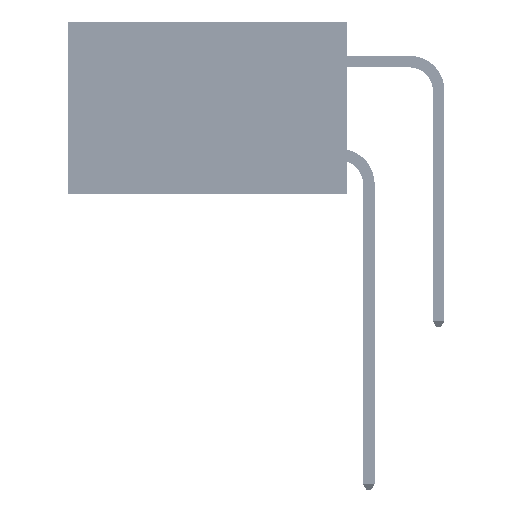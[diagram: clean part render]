
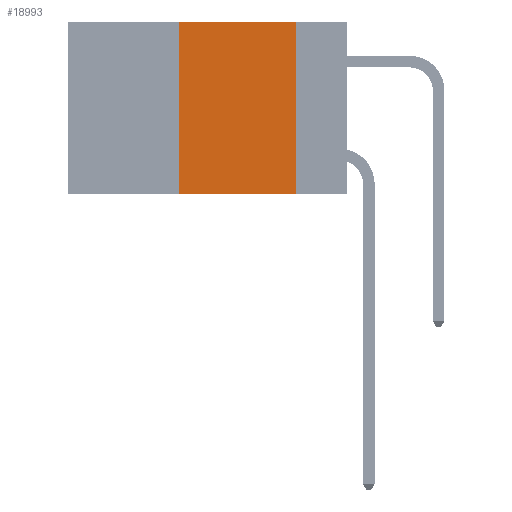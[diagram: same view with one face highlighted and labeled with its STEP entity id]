
A CAD part, left-side view. The second image highlights one B-rep face of the part: STEP entity #18993.
In plain terms, the highlighted planar face has unit normal (-1, 0, 0).
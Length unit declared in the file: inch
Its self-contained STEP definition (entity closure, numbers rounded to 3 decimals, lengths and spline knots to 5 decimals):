
#2547 = LINE ( 'NONE', #6751, #9694 ) ;
#3006 = LINE ( 'NONE', #51814, #30698 ) ;
#5474 = DIRECTION ( 'NONE',  ( 0., 0., -1. ) ) ;
#6481 = LINE ( 'NONE', #18073, #32411 ) ;
#6751 = CARTESIAN_POINT ( 'NONE',  ( 0., 0.36, 0. ) ) ;
#9428 = FACE_OUTER_BOUND ( 'NONE', #39500, .T. ) ;
#9694 = VECTOR ( 'NONE', #34959, 39.37008 ) ;
#10251 = ORIENTED_EDGE ( 'NONE', *, *, #39756, .F. ) ;
#11945 = CARTESIAN_POINT ( 'NONE',  ( 0., 0.6, 0. ) ) ;
#12634 = ORIENTED_EDGE ( 'NONE', *, *, #43634, .F. ) ;
#14637 = DIRECTION ( 'NONE',  ( 0., -1., 0. ) ) ;
#15015 = VERTEX_POINT ( 'NONE', #19865 ) ;
#17127 = ORIENTED_EDGE ( 'NONE', *, *, #45920, .F. ) ;
#17596 = CARTESIAN_POINT ( 'NONE',  ( 0., 0.11, -0.37 ) ) ;
#18073 = CARTESIAN_POINT ( 'NONE',  ( 0., 0.11, 0. ) ) ;
#18993 = ADVANCED_FACE ( 'NONE', ( #9428 ), #22057, .F. ) ;
#19465 = VERTEX_POINT ( 'NONE', #27508 ) ;
#19540 = EDGE_CURVE ( 'NONE', #19465, #24211, #3006, .T. ) ;
#19865 = CARTESIAN_POINT ( 'NONE',  ( 0., 0.11, 0. ) ) ;
#20505 = VECTOR ( 'NONE', #14637, 39.37008 ) ;
#22057 = PLANE ( 'NONE',  #45069 ) ;
#22510 = DIRECTION ( 'NONE',  ( 0., -1., 0. ) ) ;
#24211 = VERTEX_POINT ( 'NONE', #17596 ) ;
#24819 = VERTEX_POINT ( 'NONE', #35123 ) ;
#27508 = CARTESIAN_POINT ( 'NONE',  ( 0., 0.36, -0.37 ) ) ;
#30698 = VECTOR ( 'NONE', #22510, 39.37008 ) ;
#32411 = VECTOR ( 'NONE', #38379, 39.37008 ) ;
#33678 = ORIENTED_EDGE ( 'NONE', *, *, #19540, .T. ) ;
#34959 = DIRECTION ( 'NONE',  ( 0., 0., 1. ) ) ;
#35123 = CARTESIAN_POINT ( 'NONE',  ( 0., 0.36, 0. ) ) ;
#38379 = DIRECTION ( 'NONE',  ( 0., 0., -1. ) ) ;
#39500 = EDGE_LOOP ( 'NONE', ( #12634, #10251, #17127, #33678 ) ) ;
#39756 = EDGE_CURVE ( 'NONE', #24819, #15015, #47084, .T. ) ;
#41615 = CARTESIAN_POINT ( 'NONE',  ( 0., 0.6, 0. ) ) ;
#43634 = EDGE_CURVE ( 'NONE', #15015, #24211, #6481, .T. ) ;
#45069 = AXIS2_PLACEMENT_3D ( 'NONE', #41615, #50821, #5474 ) ;
#45920 = EDGE_CURVE ( 'NONE', #19465, #24819, #2547, .T. ) ;
#47084 = LINE ( 'NONE', #11945, #20505 ) ;
#50821 = DIRECTION ( 'NONE',  ( 1., 0., 0. ) ) ;
#51814 = CARTESIAN_POINT ( 'NONE',  ( 0., 0.6, -0.37 ) ) ;
